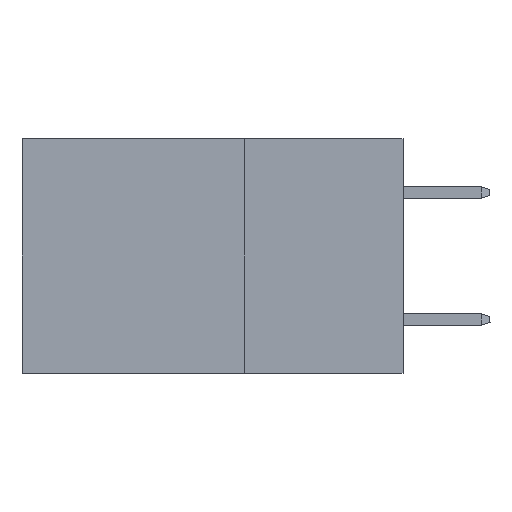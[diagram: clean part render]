
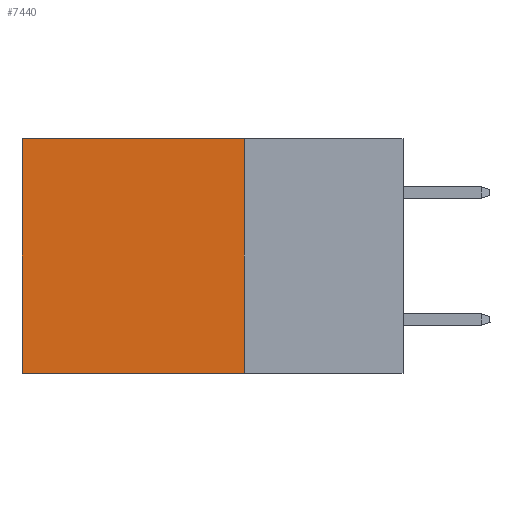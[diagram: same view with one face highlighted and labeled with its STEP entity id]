
A CAD part, left-side view. The second image highlights one B-rep face of the part: STEP entity #7440.
In plain terms, the highlighted planar face has unit normal (-1, 0, 0).
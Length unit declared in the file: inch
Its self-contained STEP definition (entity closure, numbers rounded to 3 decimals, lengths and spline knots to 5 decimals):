
#47 = CARTESIAN_POINT ( 'NONE',  ( 0.2875, 0.25, 0. ) ) ;
#98 = DIRECTION ( 'NONE',  ( 0., 0., -1. ) ) ;
#215 = FACE_OUTER_BOUND ( 'NONE', #3895, .T. ) ;
#277 = PLANE ( 'NONE',  #8424 ) ;
#416 = CARTESIAN_POINT ( 'NONE',  ( 0.2875, 0.6, 0. ) ) ;
#737 = CARTESIAN_POINT ( 'NONE',  ( 0.2875, 0.25, -0.37 ) ) ;
#914 = VERTEX_POINT ( 'NONE', #737 ) ;
#1175 = DIRECTION ( 'NONE',  ( 0., 1., 0. ) ) ;
#1526 = DIRECTION ( 'NONE',  ( 0., 0., -1. ) ) ;
#1955 = LINE ( 'NONE', #2725, #10448 ) ;
#2053 = CARTESIAN_POINT ( 'NONE',  ( 0.2875, 0.25, -0.37 ) ) ;
#2347 = VERTEX_POINT ( 'NONE', #4008 ) ;
#2725 = CARTESIAN_POINT ( 'NONE',  ( 0.2875, 0.25, 0. ) ) ;
#2989 = EDGE_CURVE ( 'NONE', #2347, #914, #11262, .T. ) ;
#3235 = CARTESIAN_POINT ( 'NONE',  ( 0.2875, 0.25, 0. ) ) ;
#3895 = EDGE_LOOP ( 'NONE', ( #10196, #9035, #11274, #5591 ) ) ;
#4008 = CARTESIAN_POINT ( 'NONE',  ( 0.2875, 0.25, 0. ) ) ;
#4111 = LINE ( 'NONE', #8518, #11389 ) ;
#4252 = VECTOR ( 'NONE', #1175, 39.37008 ) ;
#5390 = EDGE_CURVE ( 'NONE', #914, #6838, #7346, .T. ) ;
#5591 = ORIENTED_EDGE ( 'NONE', *, *, #11325, .T. ) ;
#6321 = DIRECTION ( 'NONE',  ( 0., 1., 0. ) ) ;
#6800 = EDGE_CURVE ( 'NONE', #11422, #6838, #4111, .T. ) ;
#6838 = VERTEX_POINT ( 'NONE', #9505 ) ;
#7346 = LINE ( 'NONE', #2053, #4252 ) ;
#7440 = ADVANCED_FACE ( 'NONE', ( #215 ), #277, .F. ) ;
#8424 = AXIS2_PLACEMENT_3D ( 'NONE', #47, #9972, #98 ) ;
#8518 = CARTESIAN_POINT ( 'NONE',  ( 0.2875, 0.6, 0. ) ) ;
#9035 = ORIENTED_EDGE ( 'NONE', *, *, #5390, .F. ) ;
#9505 = CARTESIAN_POINT ( 'NONE',  ( 0.2875, 0.6, -0.37 ) ) ;
#9826 = VECTOR ( 'NONE', #1526, 39.37008 ) ;
#9972 = DIRECTION ( 'NONE',  ( 1., 0., 0. ) ) ;
#10196 = ORIENTED_EDGE ( 'NONE', *, *, #6800, .T. ) ;
#10326 = DIRECTION ( 'NONE',  ( 0., 0., -1. ) ) ;
#10448 = VECTOR ( 'NONE', #6321, 39.37008 ) ;
#11262 = LINE ( 'NONE', #3235, #9826 ) ;
#11274 = ORIENTED_EDGE ( 'NONE', *, *, #2989, .F. ) ;
#11325 = EDGE_CURVE ( 'NONE', #2347, #11422, #1955, .T. ) ;
#11389 = VECTOR ( 'NONE', #10326, 39.37008 ) ;
#11422 = VERTEX_POINT ( 'NONE', #416 ) ;
